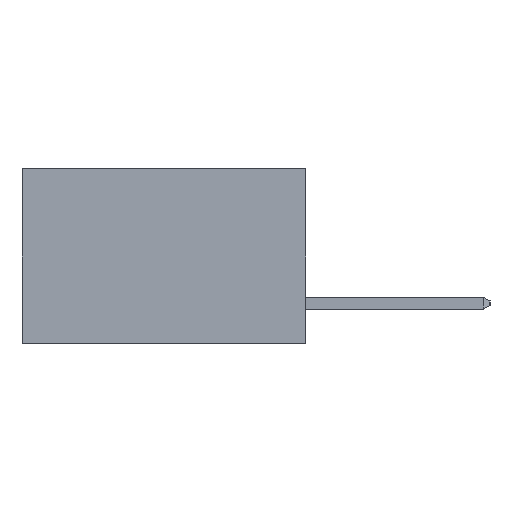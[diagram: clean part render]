
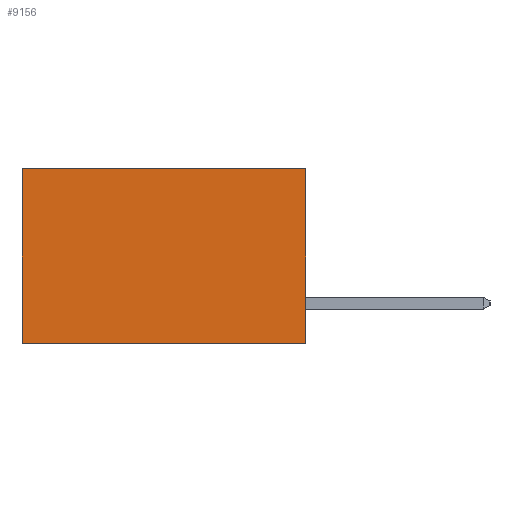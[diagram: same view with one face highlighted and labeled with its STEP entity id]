
A CAD part, left-side view. The second image highlights one B-rep face of the part: STEP entity #9156.
In plain terms, the highlighted planar face has unit normal (-1, 0, 0).
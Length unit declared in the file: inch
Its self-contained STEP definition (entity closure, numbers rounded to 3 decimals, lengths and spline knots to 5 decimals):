
#142 = ORIENTED_EDGE ( 'NONE', *, *, #6294, .F. ) ;
#283 = ORIENTED_EDGE ( 'NONE', *, *, #2074, .T. ) ;
#652 = CARTESIAN_POINT ( 'NONE',  ( 0.2615, 0.6, -0.37 ) ) ;
#2074 = EDGE_CURVE ( 'NONE', #17766, #25252, #20963, .T. ) ;
#2320 = DIRECTION ( 'NONE',  ( 0., 1., 0. ) ) ;
#2403 = CARTESIAN_POINT ( 'NONE',  ( 0.2615, 0., -0.37 ) ) ;
#2884 = ORIENTED_EDGE ( 'NONE', *, *, #23984, .T. ) ;
#2923 = EDGE_CURVE ( 'NONE', #17766, #17617, #5526, .T. ) ;
#3146 = CARTESIAN_POINT ( 'NONE',  ( 0.2615, 0., -0.37 ) ) ;
#3206 = FACE_OUTER_BOUND ( 'NONE', #25731, .T. ) ;
#5256 = ORIENTED_EDGE ( 'NONE', *, *, #2923, .F. ) ;
#5526 = LINE ( 'NONE', #3146, #25447 ) ;
#6294 = EDGE_CURVE ( 'NONE', #17617, #22718, #6956, .T. ) ;
#6359 = AXIS2_PLACEMENT_3D ( 'NONE', #19988, #21949, #9985 ) ;
#6956 = LINE ( 'NONE', #2403, #17080 ) ;
#8707 = DIRECTION ( 'NONE',  ( 0., 0., -1. ) ) ;
#9156 = ADVANCED_FACE ( 'NONE', ( #3206 ), #13961, .F. ) ;
#9985 = DIRECTION ( 'NONE',  ( 0., 0., -1. ) ) ;
#10141 = CARTESIAN_POINT ( 'NONE',  ( 0.2615, 0., -0.37 ) ) ;
#12530 = CARTESIAN_POINT ( 'NONE',  ( 0.2615, 0., 0. ) ) ;
#13961 = PLANE ( 'NONE',  #6359 ) ;
#15310 = DIRECTION ( 'NONE',  ( 0., 0., -1. ) ) ;
#16220 = CARTESIAN_POINT ( 'NONE',  ( 0.2615, 0.6, -0.37 ) ) ;
#17075 = CARTESIAN_POINT ( 'NONE',  ( 0.2615, 0.6, 0. ) ) ;
#17080 = VECTOR ( 'NONE', #2320, 39.37008 ) ;
#17617 = VERTEX_POINT ( 'NONE', #10141 ) ;
#17766 = VERTEX_POINT ( 'NONE', #12530 ) ;
#18804 = VECTOR ( 'NONE', #8707, 39.37008 ) ;
#19988 = CARTESIAN_POINT ( 'NONE',  ( 0.2615, 0., -0.37 ) ) ;
#20963 = LINE ( 'NONE', #23730, #25502 ) ;
#21949 = DIRECTION ( 'NONE',  ( 1., 0., 0. ) ) ;
#22718 = VERTEX_POINT ( 'NONE', #16220 ) ;
#23340 = LINE ( 'NONE', #652, #18804 ) ;
#23426 = DIRECTION ( 'NONE',  ( 0., 1., 0. ) ) ;
#23730 = CARTESIAN_POINT ( 'NONE',  ( 0.2615, 0., 0. ) ) ;
#23984 = EDGE_CURVE ( 'NONE', #25252, #22718, #23340, .T. ) ;
#25252 = VERTEX_POINT ( 'NONE', #17075 ) ;
#25447 = VECTOR ( 'NONE', #15310, 39.37008 ) ;
#25502 = VECTOR ( 'NONE', #23426, 39.37008 ) ;
#25731 = EDGE_LOOP ( 'NONE', ( #2884, #142, #5256, #283 ) ) ;
